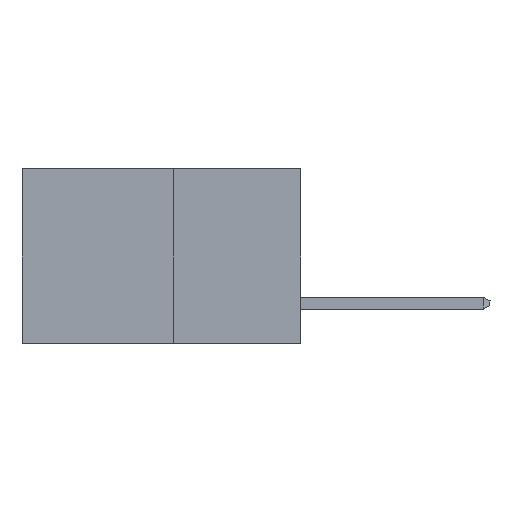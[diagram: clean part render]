
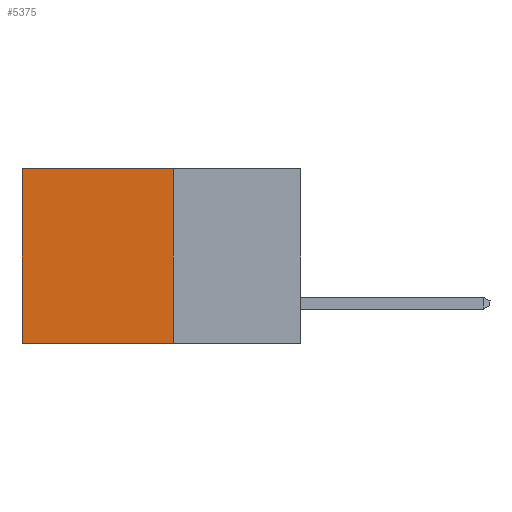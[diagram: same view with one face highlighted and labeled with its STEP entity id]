
A CAD part, left-side view. The second image highlights one B-rep face of the part: STEP entity #5375.
In plain terms, the highlighted planar face has unit normal (-1, 0, 0).
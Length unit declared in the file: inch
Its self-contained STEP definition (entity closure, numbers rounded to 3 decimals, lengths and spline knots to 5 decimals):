
#554 = DIRECTION ( 'NONE',  ( 0., 0., -1. ) ) ;
#753 = CARTESIAN_POINT ( 'NONE',  ( 0.277, 0.59, -0.37 ) ) ;
#997 = EDGE_CURVE ( 'NONE', #18251, #1139, #13165, .T. ) ;
#1089 = VECTOR ( 'NONE', #1971, 39.37008 ) ;
#1139 = VERTEX_POINT ( 'NONE', #16483 ) ;
#1463 = AXIS2_PLACEMENT_3D ( 'NONE', #13091, #12461, #12263 ) ;
#1971 = DIRECTION ( 'NONE',  ( 0., 1., 0. ) ) ;
#2305 = ORIENTED_EDGE ( 'NONE', *, *, #15862, .F. ) ;
#2551 = EDGE_LOOP ( 'NONE', ( #12757, #5531, #2305, #7982 ) ) ;
#2821 = LINE ( 'NONE', #3122, #18642 ) ;
#3122 = CARTESIAN_POINT ( 'NONE',  ( 0.277, 0.27, -0.37 ) ) ;
#3962 = CARTESIAN_POINT ( 'NONE',  ( 0.277, 0.59, 0. ) ) ;
#4293 = VERTEX_POINT ( 'NONE', #15936 ) ;
#5375 = ADVANCED_FACE ( 'NONE', ( #7860 ), #13154, .F. ) ;
#5531 = ORIENTED_EDGE ( 'NONE', *, *, #16914, .F. ) ;
#6830 = LINE ( 'NONE', #16022, #10423 ) ;
#7343 = VERTEX_POINT ( 'NONE', #18020 ) ;
#7860 = FACE_OUTER_BOUND ( 'NONE', #2551, .T. ) ;
#7982 = ORIENTED_EDGE ( 'NONE', *, *, #12964, .T. ) ;
#8453 = DIRECTION ( 'NONE',  ( 0., 0., -1. ) ) ;
#9114 = VECTOR ( 'NONE', #554, 39.37008 ) ;
#9772 = CARTESIAN_POINT ( 'NONE',  ( 0.277, 0.27, 0. ) ) ;
#10423 = VECTOR ( 'NONE', #8453, 39.37008 ) ;
#12263 = DIRECTION ( 'NONE',  ( 0., 0., -1. ) ) ;
#12430 = DIRECTION ( 'NONE',  ( 0., 1., 0. ) ) ;
#12461 = DIRECTION ( 'NONE',  ( 1., 0., 0. ) ) ;
#12757 = ORIENTED_EDGE ( 'NONE', *, *, #997, .T. ) ;
#12964 = EDGE_CURVE ( 'NONE', #7343, #18251, #13435, .T. ) ;
#13091 = CARTESIAN_POINT ( 'NONE',  ( 0.277, 0.27, -0.37 ) ) ;
#13154 = PLANE ( 'NONE',  #1463 ) ;
#13165 = LINE ( 'NONE', #753, #9114 ) ;
#13435 = LINE ( 'NONE', #9772, #1089 ) ;
#15862 = EDGE_CURVE ( 'NONE', #7343, #4293, #6830, .T. ) ;
#15936 = CARTESIAN_POINT ( 'NONE',  ( 0.277, 0.27, -0.37 ) ) ;
#16022 = CARTESIAN_POINT ( 'NONE',  ( 0.277, 0.27, -0.37 ) ) ;
#16483 = CARTESIAN_POINT ( 'NONE',  ( 0.277, 0.59, -0.37 ) ) ;
#16914 = EDGE_CURVE ( 'NONE', #4293, #1139, #2821, .T. ) ;
#18020 = CARTESIAN_POINT ( 'NONE',  ( 0.277, 0.27, 0. ) ) ;
#18251 = VERTEX_POINT ( 'NONE', #3962 ) ;
#18642 = VECTOR ( 'NONE', #12430, 39.37008 ) ;
